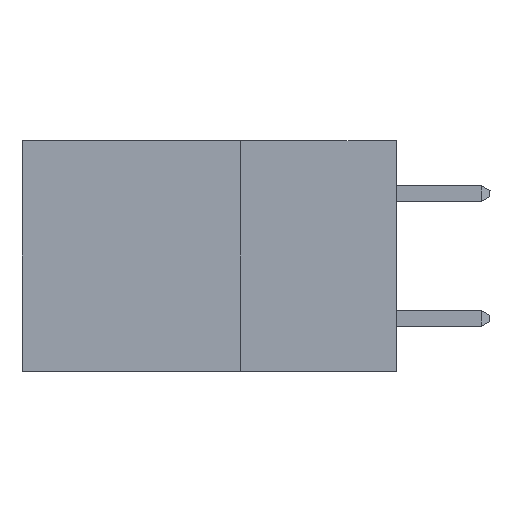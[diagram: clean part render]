
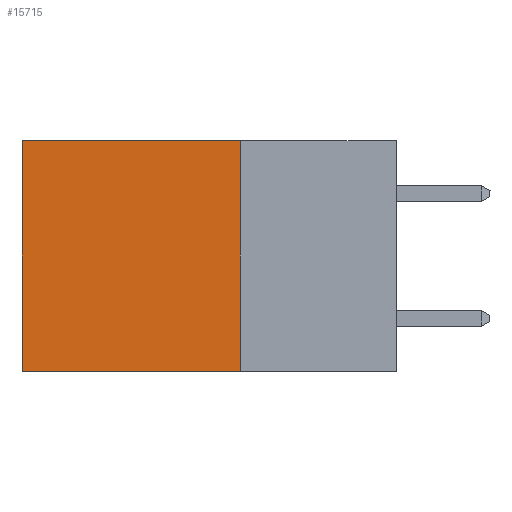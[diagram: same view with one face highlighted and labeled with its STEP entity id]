
A CAD part, left-side view. The second image highlights one B-rep face of the part: STEP entity #15715.
In plain terms, the highlighted planar face has unit normal (-1, 0, 0).
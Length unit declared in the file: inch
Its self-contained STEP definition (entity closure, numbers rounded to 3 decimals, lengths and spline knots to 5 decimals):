
#147 = LINE ( 'NONE', #20945, #4213 ) ;
#344 = DIRECTION ( 'NONE',  ( 0., 1., 0. ) ) ;
#1381 = VERTEX_POINT ( 'NONE', #17228 ) ;
#1696 = DIRECTION ( 'NONE',  ( 0., 0., -1. ) ) ;
#2123 = VERTEX_POINT ( 'NONE', #4809 ) ;
#2129 = CARTESIAN_POINT ( 'NONE',  ( 0.298, 0.6, 0. ) ) ;
#2464 = ORIENTED_EDGE ( 'NONE', *, *, #20198, .T. ) ;
#3263 = VECTOR ( 'NONE', #18823, 39.37008 ) ;
#3410 = PLANE ( 'NONE',  #8526 ) ;
#4213 = VECTOR ( 'NONE', #344, 39.37008 ) ;
#4587 = ORIENTED_EDGE ( 'NONE', *, *, #14972, .F. ) ;
#4656 = LINE ( 'NONE', #10826, #21836 ) ;
#4809 = CARTESIAN_POINT ( 'NONE',  ( 0.298, 0.6, -0.37 ) ) ;
#5734 = EDGE_CURVE ( 'NONE', #1381, #2123, #4656, .T. ) ;
#5860 = CARTESIAN_POINT ( 'NONE',  ( 0.298, 0.25, 0. ) ) ;
#6639 = LINE ( 'NONE', #8594, #10697 ) ;
#6906 = CARTESIAN_POINT ( 'NONE',  ( 0.298, 0.25, 0. ) ) ;
#8526 = AXIS2_PLACEMENT_3D ( 'NONE', #6906, #18899, #8645 ) ;
#8594 = CARTESIAN_POINT ( 'NONE',  ( 0.298, 0.25, 0. ) ) ;
#8645 = DIRECTION ( 'NONE',  ( 0., 0., -1. ) ) ;
#10697 = VECTOR ( 'NONE', #1696, 39.37008 ) ;
#10743 = DIRECTION ( 'NONE',  ( 0., 1., 0. ) ) ;
#10826 = CARTESIAN_POINT ( 'NONE',  ( 0.298, 0.25, -0.37 ) ) ;
#12468 = LINE ( 'NONE', #17082, #3263 ) ;
#13199 = ORIENTED_EDGE ( 'NONE', *, *, #17584, .T. ) ;
#13708 = VERTEX_POINT ( 'NONE', #2129 ) ;
#14972 = EDGE_CURVE ( 'NONE', #17214, #1381, #6639, .T. ) ;
#15182 = FACE_OUTER_BOUND ( 'NONE', #21151, .T. ) ;
#15715 = ADVANCED_FACE ( 'NONE', ( #15182 ), #3410, .F. ) ;
#17082 = CARTESIAN_POINT ( 'NONE',  ( 0.298, 0.6, 0. ) ) ;
#17214 = VERTEX_POINT ( 'NONE', #5860 ) ;
#17228 = CARTESIAN_POINT ( 'NONE',  ( 0.298, 0.25, -0.37 ) ) ;
#17584 = EDGE_CURVE ( 'NONE', #13708, #2123, #12468, .T. ) ;
#18823 = DIRECTION ( 'NONE',  ( 0., 0., -1. ) ) ;
#18899 = DIRECTION ( 'NONE',  ( 1., 0., 0. ) ) ;
#20198 = EDGE_CURVE ( 'NONE', #17214, #13708, #147, .T. ) ;
#20945 = CARTESIAN_POINT ( 'NONE',  ( 0.298, 0.25, 0. ) ) ;
#21151 = EDGE_LOOP ( 'NONE', ( #13199, #22166, #4587, #2464 ) ) ;
#21836 = VECTOR ( 'NONE', #10743, 39.37008 ) ;
#22166 = ORIENTED_EDGE ( 'NONE', *, *, #5734, .F. ) ;
